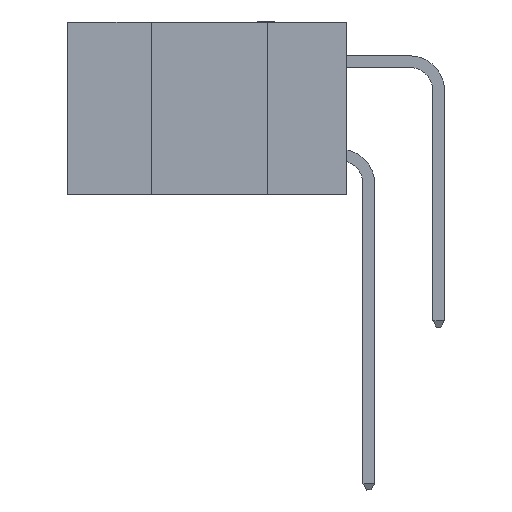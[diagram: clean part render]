
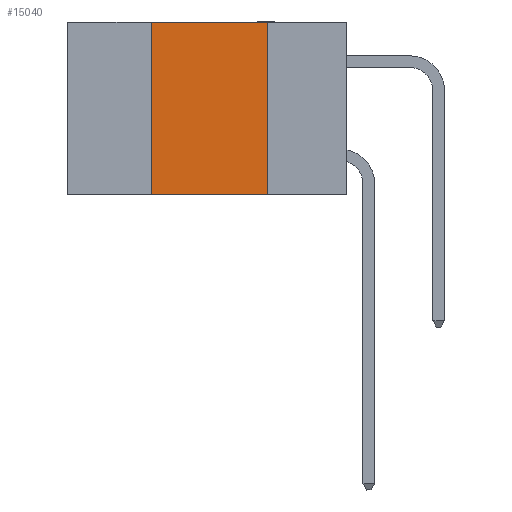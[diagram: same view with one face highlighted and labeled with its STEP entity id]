
A CAD part, left-side view. The second image highlights one B-rep face of the part: STEP entity #15040.
In plain terms, the highlighted planar face has unit normal (-1, 0, 0).
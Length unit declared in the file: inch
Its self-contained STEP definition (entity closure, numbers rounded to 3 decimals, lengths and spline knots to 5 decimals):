
#250 = EDGE_LOOP ( 'NONE', ( #19197, #34824, #29219, #30056 ) ) ;
#475 = EDGE_CURVE ( 'NONE', #8444, #22918, #29741, .T. ) ;
#954 = VERTEX_POINT ( 'NONE', #3913 ) ;
#2972 = CARTESIAN_POINT ( 'NONE',  ( 0., 0.17, -0.37 ) ) ;
#3864 = DIRECTION ( 'NONE',  ( 1., 0., 0. ) ) ;
#3913 = CARTESIAN_POINT ( 'NONE',  ( 0., 0.42, -0.37 ) ) ;
#4975 = DIRECTION ( 'NONE',  ( 0., -1., 0. ) ) ;
#5169 = DIRECTION ( 'NONE',  ( 0., 0., -1. ) ) ;
#5968 = VECTOR ( 'NONE', #19694, 39.37008 ) ;
#6258 = CARTESIAN_POINT ( 'NONE',  ( 0., 0.6, -0.37 ) ) ;
#8444 = VERTEX_POINT ( 'NONE', #16108 ) ;
#8857 = CARTESIAN_POINT ( 'NONE',  ( 0., 0.17, 0. ) ) ;
#10243 = VECTOR ( 'NONE', #5169, 39.37008 ) ;
#15040 = ADVANCED_FACE ( 'NONE', ( #32322 ), #20941, .F. ) ;
#15883 = LINE ( 'NONE', #6258, #23344 ) ;
#16108 = CARTESIAN_POINT ( 'NONE',  ( 0., 0.42, 0. ) ) ;
#16328 = CARTESIAN_POINT ( 'NONE',  ( 0., 0.6, 0. ) ) ;
#16528 = CARTESIAN_POINT ( 'NONE',  ( 0., 0.17, 0. ) ) ;
#19197 = ORIENTED_EDGE ( 'NONE', *, *, #25051, .F. ) ;
#19216 = AXIS2_PLACEMENT_3D ( 'NONE', #26376, #3864, #23712 ) ;
#19694 = DIRECTION ( 'NONE',  ( 0., 0., 1. ) ) ;
#20941 = PLANE ( 'NONE',  #19216 ) ;
#22383 = VECTOR ( 'NONE', #4975, 39.37008 ) ;
#22918 = VERTEX_POINT ( 'NONE', #8857 ) ;
#23186 = DIRECTION ( 'NONE',  ( 0., -1., 0. ) ) ;
#23344 = VECTOR ( 'NONE', #23186, 39.37008 ) ;
#23712 = DIRECTION ( 'NONE',  ( 0., 0., -1. ) ) ;
#25051 = EDGE_CURVE ( 'NONE', #22918, #25206, #27813, .T. ) ;
#25206 = VERTEX_POINT ( 'NONE', #2972 ) ;
#26376 = CARTESIAN_POINT ( 'NONE',  ( 0., 0.6, 0. ) ) ;
#27560 = LINE ( 'NONE', #36415, #5968 ) ;
#27813 = LINE ( 'NONE', #16528, #10243 ) ;
#29219 = ORIENTED_EDGE ( 'NONE', *, *, #32803, .F. ) ;
#29741 = LINE ( 'NONE', #16328, #22383 ) ;
#30056 = ORIENTED_EDGE ( 'NONE', *, *, #31190, .T. ) ;
#31190 = EDGE_CURVE ( 'NONE', #954, #25206, #15883, .T. ) ;
#32322 = FACE_OUTER_BOUND ( 'NONE', #250, .T. ) ;
#32803 = EDGE_CURVE ( 'NONE', #954, #8444, #27560, .T. ) ;
#34824 = ORIENTED_EDGE ( 'NONE', *, *, #475, .F. ) ;
#36415 = CARTESIAN_POINT ( 'NONE',  ( 0., 0.42, 0. ) ) ;
